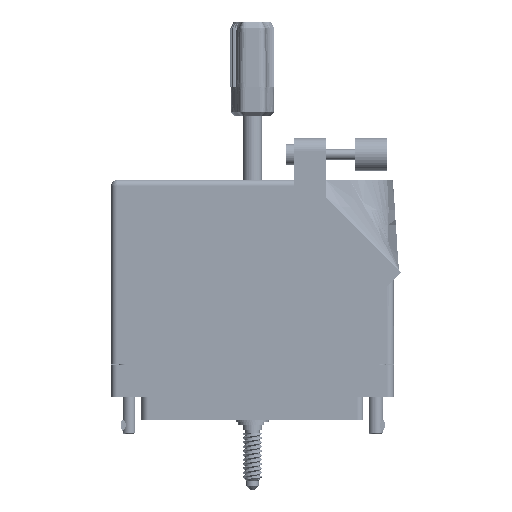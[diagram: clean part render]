
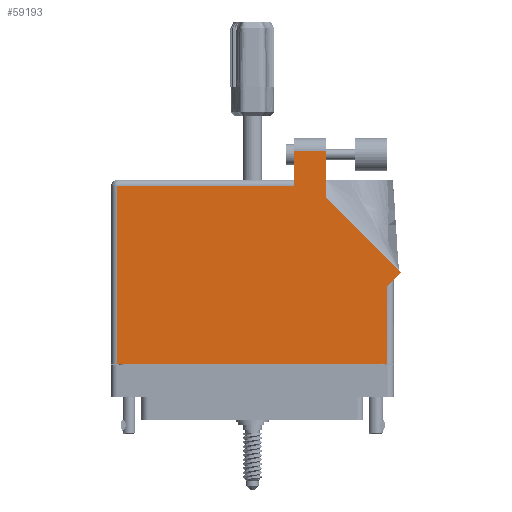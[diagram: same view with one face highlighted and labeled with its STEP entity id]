
A CAD part, front view. The second image highlights one B-rep face of the part: STEP entity #59193.
In plain terms, the highlighted face is planar.
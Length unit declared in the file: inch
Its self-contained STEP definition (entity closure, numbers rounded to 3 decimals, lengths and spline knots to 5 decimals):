
#515 = CARTESIAN_POINT ( 'NONE',  ( -1.297, 1.613, 0.617 ) ) ;
#1530 = VERTEX_POINT ( 'NONE', #51775 ) ;
#2605 = VERTEX_POINT ( 'NONE', #77344 ) ;
#3443 = CARTESIAN_POINT ( 'NONE',  ( 0.399, 1.613, 0.617 ) ) ;
#4011 = DIRECTION ( 'NONE',  ( 0.707, 0.707, 0. ) ) ;
#4427 = DIRECTION ( 'NONE',  ( -1., 0., 0. ) ) ;
#4713 = VERTEX_POINT ( 'NONE', #3443 ) ;
#7551 = VECTOR ( 'NONE', #4011, 39.37008 ) ;
#7684 = CARTESIAN_POINT ( 'NONE',  ( -1.297, -0.1, 0.617 ) ) ;
#7958 = VECTOR ( 'NONE', #31965, 39.37008 ) ;
#8469 = VECTOR ( 'NONE', #58016, 39.37008 ) ;
#8716 = EDGE_CURVE ( 'NONE', #4713, #23691, #36555, .T. ) ;
#12160 = CARTESIAN_POINT ( 'NONE',  ( -1.297, -0.1, 0.617 ) ) ;
#13770 = VECTOR ( 'NONE', #60688, 39.37008 ) ;
#14036 = EDGE_LOOP ( 'NONE', ( #53501, #37518, #24180, #72055, #92210, #82259, #16312, #55439, #15965 ) ) ;
#14113 = VECTOR ( 'NONE', #73531, 39.37008 ) ;
#14615 = CARTESIAN_POINT ( 'NONE',  ( 1.42971, 0.78571, 0.617 ) ) ;
#15965 = ORIENTED_EDGE ( 'NONE', *, *, #91348, .T. ) ;
#16312 = ORIENTED_EDGE ( 'NONE', *, *, #54054, .T. ) ;
#17285 = LINE ( 'NONE', #19192, #19624 ) ;
#17535 = AXIS2_PLACEMENT_3D ( 'NONE', #63990, #20066, #4427 ) ;
#18071 = VERTEX_POINT ( 'NONE', #14615 ) ;
#18877 = VERTEX_POINT ( 'NONE', #7684 ) ;
#19192 = CARTESIAN_POINT ( 'NONE',  ( 1.297, 0.715, 0.617 ) ) ;
#19624 = VECTOR ( 'NONE', #86297, 39.37008 ) ;
#20066 = DIRECTION ( 'NONE',  ( 0., 0., -1. ) ) ;
#21114 = CARTESIAN_POINT ( 'NONE',  ( 0.399, 1.675, 0.617 ) ) ;
#22395 = DIRECTION ( 'NONE',  ( -1., 0., 0. ) ) ;
#22990 = CARTESIAN_POINT ( 'NONE',  ( -1.359, -0.1, 0.617 ) ) ;
#23691 = VERTEX_POINT ( 'NONE', #515 ) ;
#24180 = ORIENTED_EDGE ( 'NONE', *, *, #25170, .T. ) ;
#24560 = VECTOR ( 'NONE', #22395, 39.37008 ) ;
#25170 = EDGE_CURVE ( 'NONE', #2605, #4713, #76147, .T. ) ;
#25201 = EDGE_CURVE ( 'NONE', #85054, #2605, #31635, .T. ) ;
#26199 = CARTESIAN_POINT ( 'NONE',  ( 1.359, 0.715, 0.617 ) ) ;
#31635 = LINE ( 'NONE', #67276, #24560 ) ;
#31965 = DIRECTION ( 'NONE',  ( 0., 1., 0. ) ) ;
#33167 = LINE ( 'NONE', #12160, #37870 ) ;
#34571 = CARTESIAN_POINT ( 'NONE',  ( 0.706, 1.95, 0.617 ) ) ;
#35699 = EDGE_CURVE ( 'NONE', #18877, #59931, #37221, .T. ) ;
#36555 = LINE ( 'NONE', #50472, #8469 ) ;
#37221 = LINE ( 'NONE', #22990, #13770 ) ;
#37518 = ORIENTED_EDGE ( 'NONE', *, *, #25201, .T. ) ;
#37870 = VECTOR ( 'NONE', #50147, 39.37008 ) ;
#38386 = LINE ( 'NONE', #91569, #7958 ) ;
#38584 = EDGE_CURVE ( 'NONE', #1530, #18071, #69677, .T. ) ;
#41677 = PLANE ( 'NONE',  #17535 ) ;
#43744 = CARTESIAN_POINT ( 'NONE',  ( 1.42971, 0.78571, 0.617 ) ) ;
#50147 = DIRECTION ( 'NONE',  ( 0., -1., 0. ) ) ;
#50472 = CARTESIAN_POINT ( 'NONE',  ( -1.359, 1.613, 0.617 ) ) ;
#51775 = CARTESIAN_POINT ( 'NONE',  ( 1.297, 0.653, 0.617 ) ) ;
#53501 = ORIENTED_EDGE ( 'NONE', *, *, #75559, .T. ) ;
#54054 = EDGE_CURVE ( 'NONE', #59931, #1530, #17285, .T. ) ;
#54056 = CARTESIAN_POINT ( 'NONE',  ( 1.297, -0.1, 0.617 ) ) ;
#55439 = ORIENTED_EDGE ( 'NONE', *, *, #38584, .T. ) ;
#58016 = DIRECTION ( 'NONE',  ( -1., 0., 0. ) ) ;
#59193 = ADVANCED_FACE ( 'NONE', ( #83006 ), #41677, .F. ) ;
#59931 = VERTEX_POINT ( 'NONE', #54056 ) ;
#60688 = DIRECTION ( 'NONE',  ( 1., 0., 0. ) ) ;
#63036 = VECTOR ( 'NONE', #66400, 39.37008 ) ;
#63990 = CARTESIAN_POINT ( 'NONE',  ( -1.359, 1.675, 0.617 ) ) ;
#66400 = DIRECTION ( 'NONE',  ( -0.707, 0.707, 0. ) ) ;
#67276 = CARTESIAN_POINT ( 'NONE',  ( 0.399, 1.95, 0.617 ) ) ;
#69677 = LINE ( 'NONE', #26199, #7551 ) ;
#72055 = ORIENTED_EDGE ( 'NONE', *, *, #8716, .T. ) ;
#73531 = DIRECTION ( 'NONE',  ( 0., -1., 0. ) ) ;
#75559 = EDGE_CURVE ( 'NONE', #91560, #85054, #38386, .T. ) ;
#76147 = LINE ( 'NONE', #21114, #14113 ) ;
#77344 = CARTESIAN_POINT ( 'NONE',  ( 0.399, 1.95, 0.617 ) ) ;
#77943 = CARTESIAN_POINT ( 'NONE',  ( 0.706, 1.50942, 0.617 ) ) ;
#82259 = ORIENTED_EDGE ( 'NONE', *, *, #35699, .T. ) ;
#82932 = EDGE_CURVE ( 'NONE', #23691, #18877, #33167, .T. ) ;
#83006 = FACE_OUTER_BOUND ( 'NONE', #14036, .T. ) ;
#85054 = VERTEX_POINT ( 'NONE', #34571 ) ;
#86297 = DIRECTION ( 'NONE',  ( 0., 1., 0. ) ) ;
#87557 = LINE ( 'NONE', #43744, #63036 ) ;
#91348 = EDGE_CURVE ( 'NONE', #18071, #91560, #87557, .T. ) ;
#91560 = VERTEX_POINT ( 'NONE', #77943 ) ;
#91569 = CARTESIAN_POINT ( 'NONE',  ( 0.706, 1.50942, 0.617 ) ) ;
#92210 = ORIENTED_EDGE ( 'NONE', *, *, #82932, .T. ) ;
